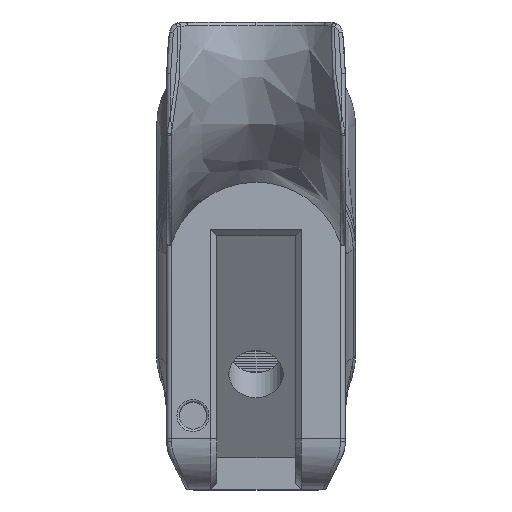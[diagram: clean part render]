
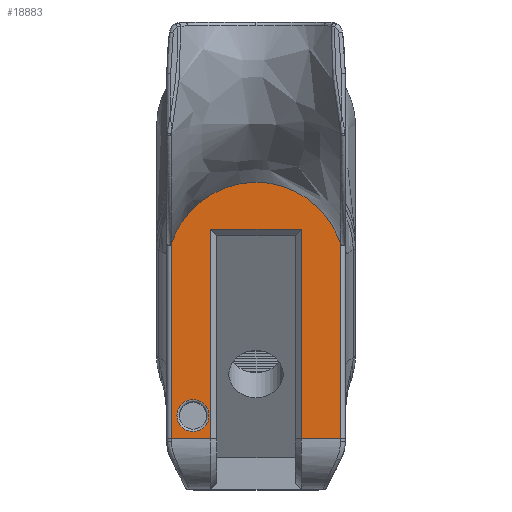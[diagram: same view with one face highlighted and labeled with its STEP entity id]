
A CAD part, top view. The second image highlights one B-rep face of the part: STEP entity #18883.
In plain terms, the highlighted planar face has unit normal (0, 0, 1).
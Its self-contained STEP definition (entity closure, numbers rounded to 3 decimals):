
#236=FACE_BOUND('',#5206,.T.);
#941=PLANE('',#20473);
#1444=LINE('',#40739,#2513);
#1482=LINE('',#42439,#2551);
#1483=LINE('',#42443,#2552);
#1818=LINE('',#45280,#2887);
#1819=LINE('',#45282,#2888);
#1820=LINE('',#45284,#2889);
#1821=LINE('',#45285,#2890);
#2513=VECTOR('',#22278,10.);
#2551=VECTOR('',#22458,10.);
#2552=VECTOR('',#22463,10.);
#2887=VECTOR('',#24350,10.);
#2888=VECTOR('',#24351,10.);
#2889=VECTOR('',#24352,10.);
#2890=VECTOR('',#24353,10.);
#4003=FACE_OUTER_BOUND('',#5205,.T.);
#5205=EDGE_LOOP('',(#16117,#16118,#16119,#16120,#16121,#16122,#16123,#16124,
#16125));
#5206=EDGE_LOOP('',(#16126));
#6189=B_SPLINE_CURVE_WITH_KNOTS('',3,(#45223,#45224,#45225,#45226,#45227,
#45228,#45229,#45230,#45231,#45232),.UNSPECIFIED.,.F.,.F.,(4,2,2,2,4),(3.835,
4.196,4.64,5.076,5.232),
 .UNSPECIFIED.);
#6196=B_SPLINE_CURVE_WITH_KNOTS('',3,(#45268,#45269,#45270,#45271,#45272,
#45273,#45274,#45275,#45276,#45277),.UNSPECIFIED.,.F.,.F.,(4,2,2,2,4),(5.232,
5.504,5.934,6.283,6.628),
 .UNSPECIFIED.);
#6456=CIRCLE('',#19638,2.);
#8033=VERTEX_POINT('',#40736);
#8034=VERTEX_POINT('',#40738);
#8045=VERTEX_POINT('',#40778);
#8126=VERTEX_POINT('',#42429);
#8129=VERTEX_POINT('',#42442);
#8579=VERTEX_POINT('',#45221);
#8580=VERTEX_POINT('',#45222);
#8586=VERTEX_POINT('',#45279);
#8587=VERTEX_POINT('',#45281);
#8588=VERTEX_POINT('',#45283);
#10184=EDGE_CURVE('',#8034,#8033,#1444,.T.);
#10202=EDGE_CURVE('',#8045,#8045,#6456,.T.);
#10344=EDGE_CURVE('',#8126,#8034,#1482,.T.);
#10346=EDGE_CURVE('',#8126,#8129,#1483,.T.);
#11157=EDGE_CURVE('',#8579,#8580,#6189,.F.);
#11164=EDGE_CURVE('',#8129,#8579,#6196,.F.);
#11165=EDGE_CURVE('',#8586,#8033,#1818,.T.);
#11166=EDGE_CURVE('',#8587,#8586,#1819,.T.);
#11167=EDGE_CURVE('',#8588,#8587,#1820,.T.);
#11168=EDGE_CURVE('',#8580,#8588,#1821,.T.);
#16117=ORIENTED_EDGE('',*,*,#11165,.F.);
#16118=ORIENTED_EDGE('',*,*,#11166,.F.);
#16119=ORIENTED_EDGE('',*,*,#11167,.F.);
#16120=ORIENTED_EDGE('',*,*,#11168,.F.);
#16121=ORIENTED_EDGE('',*,*,#11157,.F.);
#16122=ORIENTED_EDGE('',*,*,#11164,.F.);
#16123=ORIENTED_EDGE('',*,*,#10346,.F.);
#16124=ORIENTED_EDGE('',*,*,#10344,.T.);
#16125=ORIENTED_EDGE('',*,*,#10184,.T.);
#16126=ORIENTED_EDGE('',*,*,#10202,.F.);
#18883=ADVANCED_FACE('',(#4003,#236),#941,.T.);
#19638=AXIS2_PLACEMENT_3D('',#40779,#22316,#22317);
#20473=AXIS2_PLACEMENT_3D('',#45278,#24348,#24349);
#22278=DIRECTION('',(0.,1.,0.));
#22316=DIRECTION('center_axis',(0.,0.,
1.));
#22317=DIRECTION('ref_axis',(-1.,0.,0.));
#22458=DIRECTION('',(1.,0.,0.));
#22463=DIRECTION('',(0.,1.,0.));
#24348=DIRECTION('center_axis',(0.,0.,
1.));
#24349=DIRECTION('ref_axis',(0.,-1.,0.));
#24350=DIRECTION('',(-1.,0.,0.));
#24351=DIRECTION('',(0.,1.,0.));
#24352=DIRECTION('',(-1.,0.,0.));
#24353=DIRECTION('',(0.,-1.,0.));
#40736=CARTESIAN_POINT('',(18.417,-117.318,28.406));
#40738=CARTESIAN_POINT('',(18.417,-143.468,28.406));
#40739=CARTESIAN_POINT('',(18.417,-114.618,28.406));
#40778=CARTESIAN_POINT('',(18.205,-140.572,28.406));
#40779=CARTESIAN_POINT('Origin',(16.205,-140.572,28.406));
#42429=CARTESIAN_POINT('',(13.518,-143.468,28.406));
#42439=CARTESIAN_POINT('',(28.956,-143.468,28.406));
#42442=CARTESIAN_POINT('',(13.518,-119.074,28.406));
#42443=CARTESIAN_POINT('',(13.518,-40.367,28.406));
#45221=CARTESIAN_POINT('',(24.081,-111.416,28.406));
#45222=CARTESIAN_POINT('',(34.645,-119.074,28.406));
#45223=CARTESIAN_POINT('Ctrl Pts',(34.645,-119.074,28.406));
#45224=CARTESIAN_POINT('Ctrl Pts',(34.258,-117.938,28.406));
#45225=CARTESIAN_POINT('Ctrl Pts',(33.695,-116.869,28.406));
#45226=CARTESIAN_POINT('Ctrl Pts',(32.086,-114.722,28.406));
#45227=CARTESIAN_POINT('Ctrl Pts',(30.975,-113.721,28.406));
#45228=CARTESIAN_POINT('Ctrl Pts',(28.452,-112.223,28.406));
#45229=CARTESIAN_POINT('Ctrl Pts',(27.068,-111.732,28.406));
#45230=CARTESIAN_POINT('Ctrl Pts',(25.114,-111.452,28.406));
#45231=CARTESIAN_POINT('Ctrl Pts',(24.598,-111.416,28.406));
#45232=CARTESIAN_POINT('Ctrl Pts',(24.081,-111.416,28.406));
#45268=CARTESIAN_POINT('Ctrl Pts',(24.081,-111.416,28.406));
#45269=CARTESIAN_POINT('Ctrl Pts',(23.179,-111.416,28.406));
#45270=CARTESIAN_POINT('Ctrl Pts',(22.278,-111.528,28.406));
#45271=CARTESIAN_POINT('Ctrl Pts',(20.011,-112.101,28.406));
#45272=CARTESIAN_POINT('Ctrl Pts',(18.705,-112.72,28.406));
#45273=CARTESIAN_POINT('Ctrl Pts',(16.612,-114.256,28.406));
#45274=CARTESIAN_POINT('Ctrl Pts',(15.785,-115.087,28.406));
#45275=CARTESIAN_POINT('Ctrl Pts',(14.422,-116.958,28.406));
#45276=CARTESIAN_POINT('Ctrl Pts',(13.889,-117.985,28.406));
#45277=CARTESIAN_POINT('Ctrl Pts',(13.518,-119.074,28.406));
#45278=CARTESIAN_POINT('Origin',(19.207,-112.624,28.406));
#45279=CARTESIAN_POINT('',(29.746,-117.318,28.406));
#45280=CARTESIAN_POINT('',(24.173,-117.318,28.406));
#45281=CARTESIAN_POINT('',(29.746,-143.468,28.406));
#45282=CARTESIAN_POINT('',(29.746,-114.618,28.406));
#45283=CARTESIAN_POINT('',(34.645,-143.468,28.406));
#45284=CARTESIAN_POINT('',(19.207,-143.468,28.406));
#45285=CARTESIAN_POINT('',(34.645,-40.367,28.406));
